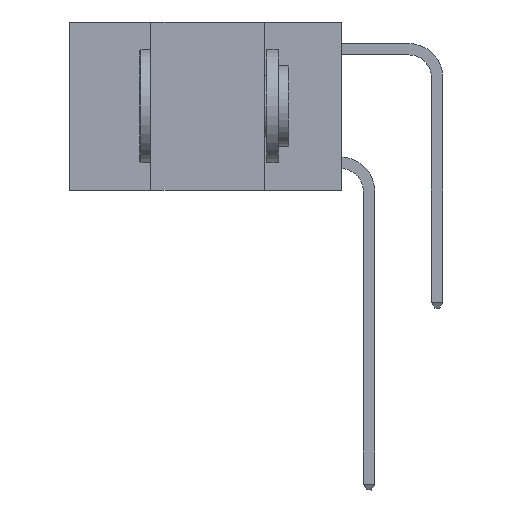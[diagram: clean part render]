
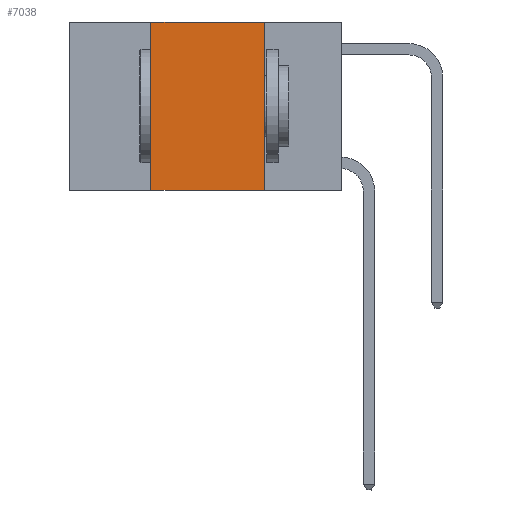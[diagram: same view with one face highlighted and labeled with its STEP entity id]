
A CAD part, left-side view. The second image highlights one B-rep face of the part: STEP entity #7038.
In plain terms, the highlighted planar face has unit normal (-1, 0, 0).
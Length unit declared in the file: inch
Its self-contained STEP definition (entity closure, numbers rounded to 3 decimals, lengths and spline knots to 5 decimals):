
#92 = CARTESIAN_POINT ( 'NONE',  ( 0., 0.6, 0. ) ) ;
#1050 = EDGE_CURVE ( 'NONE', #3976, #10719, #27670, .T. ) ;
#1162 = CARTESIAN_POINT ( 'NONE',  ( 0., 0.6, -0.37 ) ) ;
#2050 = PLANE ( 'NONE',  #10313 ) ;
#2700 = EDGE_CURVE ( 'NONE', #10719, #15572, #4401, .T. ) ;
#3976 = VERTEX_POINT ( 'NONE', #21681 ) ;
#4401 = LINE ( 'NONE', #17654, #14899 ) ;
#5283 = VERTEX_POINT ( 'NONE', #16048 ) ;
#7038 = ADVANCED_FACE ( 'NONE', ( #11741 ), #2050, .F. ) ;
#7355 = VECTOR ( 'NONE', #13178, 39.37008 ) ;
#9210 = LINE ( 'NONE', #16425, #22406 ) ;
#10313 = AXIS2_PLACEMENT_3D ( 'NONE', #25278, #11422, #13576 ) ;
#10719 = VERTEX_POINT ( 'NONE', #20478 ) ;
#11422 = DIRECTION ( 'NONE',  ( 1., 0., 0. ) ) ;
#11496 = ORIENTED_EDGE ( 'NONE', *, *, #2700, .F. ) ;
#11741 = FACE_OUTER_BOUND ( 'NONE', #26700, .T. ) ;
#12899 = EDGE_CURVE ( 'NONE', #5283, #15572, #14999, .T. ) ;
#12961 = CARTESIAN_POINT ( 'NONE',  ( 0., 0.17, -0.37 ) ) ;
#13178 = DIRECTION ( 'NONE',  ( 0., -1., 0. ) ) ;
#13206 = DIRECTION ( 'NONE',  ( 0., 0., -1. ) ) ;
#13576 = DIRECTION ( 'NONE',  ( 0., 0., -1. ) ) ;
#14899 = VECTOR ( 'NONE', #13206, 39.37008 ) ;
#14999 = LINE ( 'NONE', #1162, #7355 ) ;
#15572 = VERTEX_POINT ( 'NONE', #12961 ) ;
#15810 = VECTOR ( 'NONE', #26407, 39.37008 ) ;
#16048 = CARTESIAN_POINT ( 'NONE',  ( 0., 0.42, -0.37 ) ) ;
#16425 = CARTESIAN_POINT ( 'NONE',  ( 0., 0.42, 0. ) ) ;
#17654 = CARTESIAN_POINT ( 'NONE',  ( 0., 0.17, 0. ) ) ;
#17734 = ORIENTED_EDGE ( 'NONE', *, *, #1050, .F. ) ;
#20478 = CARTESIAN_POINT ( 'NONE',  ( 0., 0.17, 0. ) ) ;
#21681 = CARTESIAN_POINT ( 'NONE',  ( 0., 0.42, 0. ) ) ;
#22406 = VECTOR ( 'NONE', #25692, 39.37008 ) ;
#22830 = ORIENTED_EDGE ( 'NONE', *, *, #29552, .F. ) ;
#24794 = ORIENTED_EDGE ( 'NONE', *, *, #12899, .T. ) ;
#25278 = CARTESIAN_POINT ( 'NONE',  ( 0., 0.6, 0. ) ) ;
#25692 = DIRECTION ( 'NONE',  ( 0., 0., 1. ) ) ;
#26407 = DIRECTION ( 'NONE',  ( 0., -1., 0. ) ) ;
#26700 = EDGE_LOOP ( 'NONE', ( #11496, #17734, #22830, #24794 ) ) ;
#27670 = LINE ( 'NONE', #92, #15810 ) ;
#29552 = EDGE_CURVE ( 'NONE', #5283, #3976, #9210, .T. ) ;
